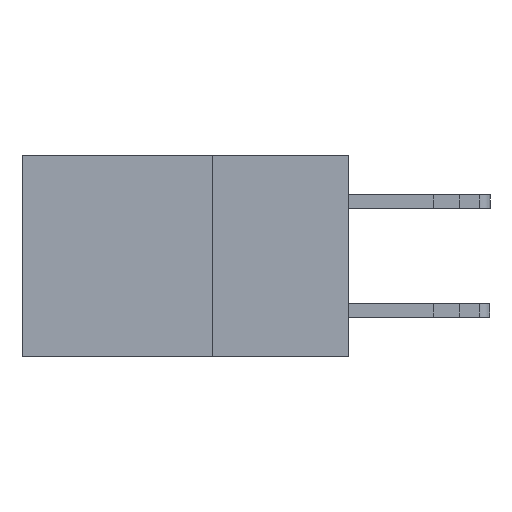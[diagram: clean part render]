
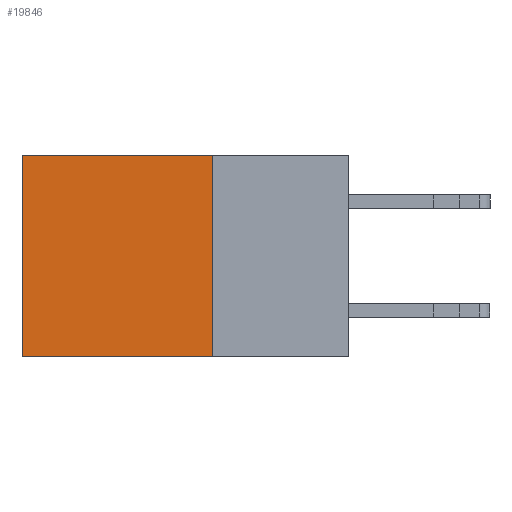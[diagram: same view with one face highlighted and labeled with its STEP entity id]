
A CAD part, left-side view. The second image highlights one B-rep face of the part: STEP entity #19846.
In plain terms, the highlighted planar face has unit normal (-1, 0, 0).
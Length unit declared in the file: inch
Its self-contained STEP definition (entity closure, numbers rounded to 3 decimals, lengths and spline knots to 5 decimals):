
#47 = CARTESIAN_POINT ( 'NONE',  ( 0.298, 0.25, 0. ) ) ;
#404 = CARTESIAN_POINT ( 'NONE',  ( 0.298, 0.6, -0.37 ) ) ;
#756 = EDGE_CURVE ( 'NONE', #17045, #23693, #12077, .T. ) ;
#1974 = DIRECTION ( 'NONE',  ( 0., 1., 0. ) ) ;
#3722 = VERTEX_POINT ( 'NONE', #13285 ) ;
#3852 = CARTESIAN_POINT ( 'NONE',  ( 0.298, 0.6, 0. ) ) ;
#4463 = VECTOR ( 'NONE', #1974, 39.37008 ) ;
#6470 = ORIENTED_EDGE ( 'NONE', *, *, #19208, .F. ) ;
#6687 = DIRECTION ( 'NONE',  ( 0., 0., -1. ) ) ;
#7159 = CARTESIAN_POINT ( 'NONE',  ( 0.298, 0.25, 0. ) ) ;
#7902 = VECTOR ( 'NONE', #13417, 39.37008 ) ;
#10119 = LINE ( 'NONE', #47, #4463 ) ;
#10814 = ORIENTED_EDGE ( 'NONE', *, *, #22196, .T. ) ;
#10826 = CARTESIAN_POINT ( 'NONE',  ( 0.298, 0.25, -0.37 ) ) ;
#10965 = DIRECTION ( 'NONE',  ( 0., 0., -1. ) ) ;
#12077 = LINE ( 'NONE', #16402, #21625 ) ;
#12912 = LINE ( 'NONE', #3852, #7902 ) ;
#12993 = AXIS2_PLACEMENT_3D ( 'NONE', #7159, #22356, #10965 ) ;
#13285 = CARTESIAN_POINT ( 'NONE',  ( 0.298, 0.25, 0. ) ) ;
#13417 = DIRECTION ( 'NONE',  ( 0., 0., -1. ) ) ;
#13512 = LINE ( 'NONE', #18011, #23035 ) ;
#13991 = VERTEX_POINT ( 'NONE', #23575 ) ;
#15679 = EDGE_CURVE ( 'NONE', #13991, #23693, #12912, .T. ) ;
#15904 = FACE_OUTER_BOUND ( 'NONE', #22943, .T. ) ;
#16402 = CARTESIAN_POINT ( 'NONE',  ( 0.298, 0.25, -0.37 ) ) ;
#17012 = ORIENTED_EDGE ( 'NONE', *, *, #756, .F. ) ;
#17045 = VERTEX_POINT ( 'NONE', #10826 ) ;
#18011 = CARTESIAN_POINT ( 'NONE',  ( 0.298, 0.25, 0. ) ) ;
#19208 = EDGE_CURVE ( 'NONE', #3722, #17045, #13512, .T. ) ;
#19846 = ADVANCED_FACE ( 'NONE', ( #15904 ), #24189, .F. ) ;
#19890 = DIRECTION ( 'NONE',  ( 0., 1., 0. ) ) ;
#21434 = ORIENTED_EDGE ( 'NONE', *, *, #15679, .T. ) ;
#21625 = VECTOR ( 'NONE', #19890, 39.37008 ) ;
#22196 = EDGE_CURVE ( 'NONE', #3722, #13991, #10119, .T. ) ;
#22356 = DIRECTION ( 'NONE',  ( 1., 0., 0. ) ) ;
#22943 = EDGE_LOOP ( 'NONE', ( #21434, #17012, #6470, #10814 ) ) ;
#23035 = VECTOR ( 'NONE', #6687, 39.37008 ) ;
#23575 = CARTESIAN_POINT ( 'NONE',  ( 0.298, 0.6, 0. ) ) ;
#23693 = VERTEX_POINT ( 'NONE', #404 ) ;
#24189 = PLANE ( 'NONE',  #12993 ) ;
